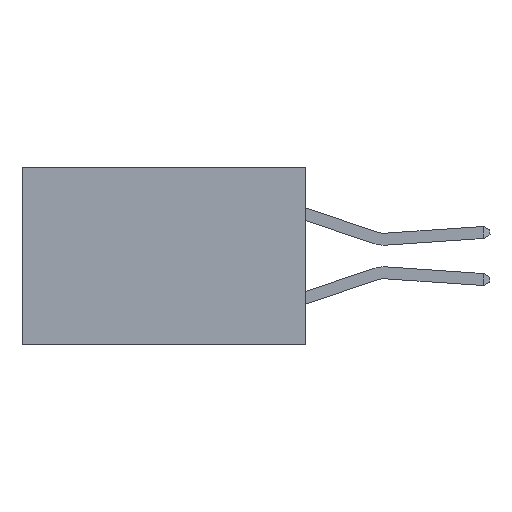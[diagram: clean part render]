
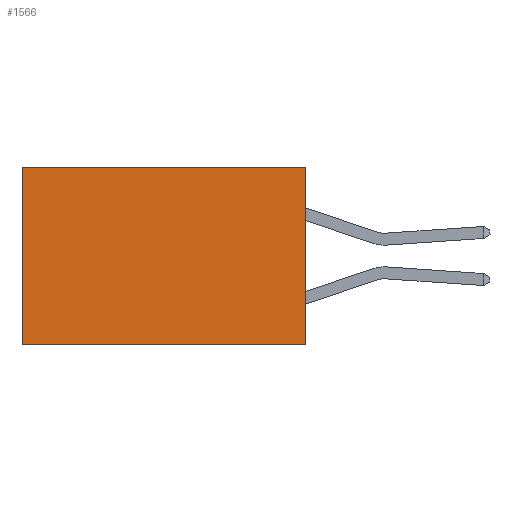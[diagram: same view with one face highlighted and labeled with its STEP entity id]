
A CAD part, left-side view. The second image highlights one B-rep face of the part: STEP entity #1566.
In plain terms, the highlighted planar face has unit normal (-1, 0, 0).
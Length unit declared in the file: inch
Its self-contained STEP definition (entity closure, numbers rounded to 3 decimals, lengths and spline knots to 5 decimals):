
#122 = LINE ( 'NONE', #5978, #6634 ) ;
#833 = EDGE_LOOP ( 'NONE', ( #2054, #3597, #8571, #8707 ) ) ;
#1223 = DIRECTION ( 'NONE',  ( 0., 1., 0. ) ) ;
#1274 = VERTEX_POINT ( 'NONE', #4971 ) ;
#1566 = ADVANCED_FACE ( 'NONE', ( #6971 ), #2958, .F. ) ;
#1759 = EDGE_CURVE ( 'NONE', #9452, #1274, #122, .T. ) ;
#2032 = EDGE_CURVE ( 'NONE', #1274, #8847, #7508, .T. ) ;
#2054 = ORIENTED_EDGE ( 'NONE', *, *, #2032, .T. ) ;
#2301 = LINE ( 'NONE', #7379, #4354 ) ;
#2408 = AXIS2_PLACEMENT_3D ( 'NONE', #8509, #6189, #8262 ) ;
#2621 = VECTOR ( 'NONE', #4883, 39.37008 ) ;
#2958 = PLANE ( 'NONE',  #2408 ) ;
#3597 = ORIENTED_EDGE ( 'NONE', *, *, #4451, .F. ) ;
#3815 = EDGE_CURVE ( 'NONE', #9452, #4935, #8701, .T. ) ;
#4354 = VECTOR ( 'NONE', #8585, 39.37008 ) ;
#4451 = EDGE_CURVE ( 'NONE', #4935, #8847, #2301, .T. ) ;
#4819 = DIRECTION ( 'NONE',  ( 0., 0., -1. ) ) ;
#4883 = DIRECTION ( 'NONE',  ( 0., 0., -1. ) ) ;
#4935 = VERTEX_POINT ( 'NONE', #4968 ) ;
#4968 = CARTESIAN_POINT ( 'NONE',  ( 0.277, 0., -0.37 ) ) ;
#4971 = CARTESIAN_POINT ( 'NONE',  ( 0.277, 0.59, 0. ) ) ;
#5003 = CARTESIAN_POINT ( 'NONE',  ( 0.277, 0., -0.37 ) ) ;
#5574 = VECTOR ( 'NONE', #4819, 39.37008 ) ;
#5978 = CARTESIAN_POINT ( 'NONE',  ( 0.277, 0., 0. ) ) ;
#6189 = DIRECTION ( 'NONE',  ( 1., 0., 0. ) ) ;
#6634 = VECTOR ( 'NONE', #1223, 39.37008 ) ;
#6858 = CARTESIAN_POINT ( 'NONE',  ( 0.277, 0.59, -0.37 ) ) ;
#6971 = FACE_OUTER_BOUND ( 'NONE', #833, .T. ) ;
#7379 = CARTESIAN_POINT ( 'NONE',  ( 0.277, 0., -0.37 ) ) ;
#7409 = CARTESIAN_POINT ( 'NONE',  ( 0.277, 0., 0. ) ) ;
#7508 = LINE ( 'NONE', #9763, #5574 ) ;
#8262 = DIRECTION ( 'NONE',  ( 0., 0., -1. ) ) ;
#8509 = CARTESIAN_POINT ( 'NONE',  ( 0.277, 0., -0.37 ) ) ;
#8571 = ORIENTED_EDGE ( 'NONE', *, *, #3815, .F. ) ;
#8585 = DIRECTION ( 'NONE',  ( 0., 1., 0. ) ) ;
#8701 = LINE ( 'NONE', #5003, #2621 ) ;
#8707 = ORIENTED_EDGE ( 'NONE', *, *, #1759, .T. ) ;
#8847 = VERTEX_POINT ( 'NONE', #6858 ) ;
#9452 = VERTEX_POINT ( 'NONE', #7409 ) ;
#9763 = CARTESIAN_POINT ( 'NONE',  ( 0.277, 0.59, -0.37 ) ) ;
